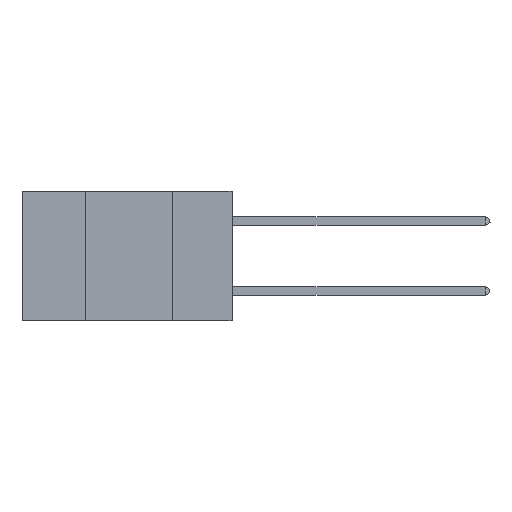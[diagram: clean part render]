
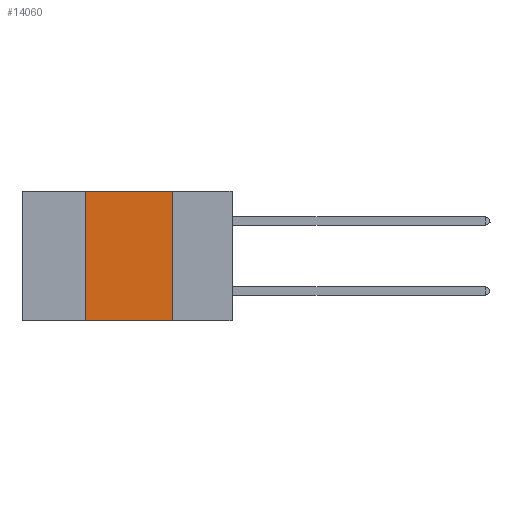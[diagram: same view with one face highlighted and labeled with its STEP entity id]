
A CAD part, left-side view. The second image highlights one B-rep face of the part: STEP entity #14060.
In plain terms, the highlighted planar face has unit normal (-1, 0, 0).
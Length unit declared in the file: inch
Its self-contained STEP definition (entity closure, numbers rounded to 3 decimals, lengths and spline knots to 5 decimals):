
#1054 = FACE_OUTER_BOUND ( 'NONE', #16426, .T. ) ;
#1763 = LINE ( 'NONE', #7517, #3698 ) ;
#1957 = ORIENTED_EDGE ( 'NONE', *, *, #2740, .F. ) ;
#2214 = CARTESIAN_POINT ( 'NONE',  ( 0., 0.17, 0. ) ) ;
#2740 = EDGE_CURVE ( 'NONE', #4633, #16392, #24488, .T. ) ;
#3698 = VECTOR ( 'NONE', #3931, 39.37008 ) ;
#3931 = DIRECTION ( 'NONE',  ( 0., -1., 0. ) ) ;
#4633 = VERTEX_POINT ( 'NONE', #2214 ) ;
#4736 = DIRECTION ( 'NONE',  ( 1., 0., 0. ) ) ;
#5547 = VERTEX_POINT ( 'NONE', #21767 ) ;
#7115 = DIRECTION ( 'NONE',  ( 0., 0., -1. ) ) ;
#7450 = LINE ( 'NONE', #22185, #25083 ) ;
#7517 = CARTESIAN_POINT ( 'NONE',  ( 0., 0.6, 0. ) ) ;
#7832 = ORIENTED_EDGE ( 'NONE', *, *, #10656, .F. ) ;
#8234 = EDGE_CURVE ( 'NONE', #5547, #16392, #7450, .T. ) ;
#8298 = VERTEX_POINT ( 'NONE', #21127 ) ;
#8575 = PLANE ( 'NONE',  #16749 ) ;
#9186 = LINE ( 'NONE', #22604, #19117 ) ;
#9775 = ORIENTED_EDGE ( 'NONE', *, *, #24292, .F. ) ;
#10656 = EDGE_CURVE ( 'NONE', #8298, #4633, #1763, .T. ) ;
#10870 = VECTOR ( 'NONE', #7115, 39.37008 ) ;
#13306 = DIRECTION ( 'NONE',  ( 0., -1., 0. ) ) ;
#14060 = ADVANCED_FACE ( 'NONE', ( #1054 ), #8575, .F. ) ;
#14546 = DIRECTION ( 'NONE',  ( 0., 0., -1. ) ) ;
#14907 = DIRECTION ( 'NONE',  ( 0., 0., 1. ) ) ;
#15242 = CARTESIAN_POINT ( 'NONE',  ( 0., 0.17, 0. ) ) ;
#16392 = VERTEX_POINT ( 'NONE', #17382 ) ;
#16426 = EDGE_LOOP ( 'NONE', ( #1957, #7832, #9775, #24680 ) ) ;
#16749 = AXIS2_PLACEMENT_3D ( 'NONE', #22128, #4736, #14546 ) ;
#17382 = CARTESIAN_POINT ( 'NONE',  ( 0., 0.17, -0.37 ) ) ;
#19117 = VECTOR ( 'NONE', #14907, 39.37008 ) ;
#21127 = CARTESIAN_POINT ( 'NONE',  ( 0., 0.42, 0. ) ) ;
#21767 = CARTESIAN_POINT ( 'NONE',  ( 0., 0.42, -0.37 ) ) ;
#22128 = CARTESIAN_POINT ( 'NONE',  ( 0., 0.6, 0. ) ) ;
#22185 = CARTESIAN_POINT ( 'NONE',  ( 0., 0.6, -0.37 ) ) ;
#22604 = CARTESIAN_POINT ( 'NONE',  ( 0., 0.42, 0. ) ) ;
#24292 = EDGE_CURVE ( 'NONE', #5547, #8298, #9186, .T. ) ;
#24488 = LINE ( 'NONE', #15242, #10870 ) ;
#24680 = ORIENTED_EDGE ( 'NONE', *, *, #8234, .T. ) ;
#25083 = VECTOR ( 'NONE', #13306, 39.37008 ) ;
